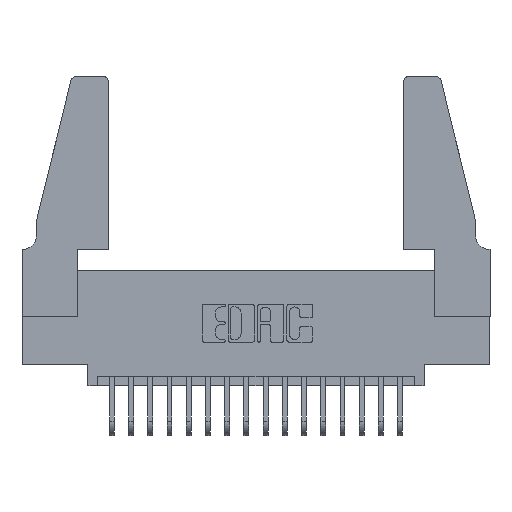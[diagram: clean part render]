
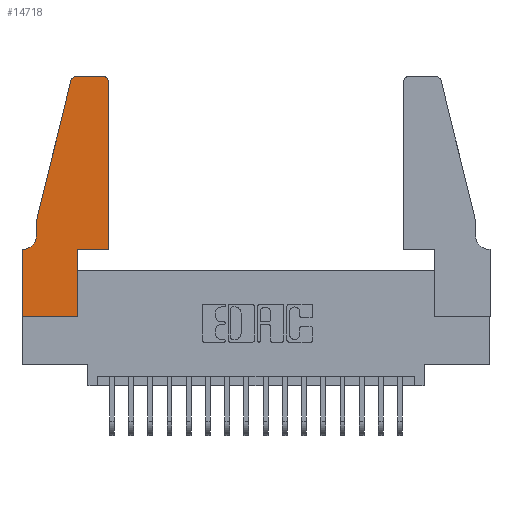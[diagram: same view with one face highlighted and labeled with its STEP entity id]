
A CAD part, top view. The second image highlights one B-rep face of the part: STEP entity #14718.
In plain terms, the highlighted planar face has unit normal (0, 0, 1).
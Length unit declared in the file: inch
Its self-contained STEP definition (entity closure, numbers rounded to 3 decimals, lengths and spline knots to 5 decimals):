
#206 = DIRECTION ( 'NONE',  ( 0., 0., -1. ) ) ;
#715 = VERTEX_POINT ( 'NONE', #1710 ) ;
#738 = DIRECTION ( 'NONE',  ( 1., 0., 0. ) ) ;
#847 = VERTEX_POINT ( 'NONE', #10963 ) ;
#925 = VECTOR ( 'NONE', #5029, 39.37008 ) ;
#1072 = CARTESIAN_POINT ( 'NONE',  ( 0.4205, 1.22, 0.37 ) ) ;
#1340 = DIRECTION ( 'NONE',  ( 0., 0., 1. ) ) ;
#1411 = VECTOR ( 'NONE', #2004, 39.37008 ) ;
#1440 = CARTESIAN_POINT ( 'NONE',  ( 0., 0., 0.37 ) ) ;
#1502 = CARTESIAN_POINT ( 'NONE',  ( 0., 0.35, 0.37 ) ) ;
#1572 = ORIENTED_EDGE ( 'NONE', *, *, #3822, .T. ) ;
#1633 = VERTEX_POINT ( 'NONE', #12237 ) ;
#1710 = CARTESIAN_POINT ( 'NONE',  ( 0., 0., 0.37 ) ) ;
#1793 = ORIENTED_EDGE ( 'NONE', *, *, #8181, .T. ) ;
#1916 = DIRECTION ( 'NONE',  ( -1., 0., 0. ) ) ;
#2004 = DIRECTION ( 'NONE',  ( -1., 0., 0. ) ) ;
#2450 = DIRECTION ( 'NONE',  ( 1., 0., 0. ) ) ;
#2582 = CIRCLE ( 'NONE', #15649, 0.03 ) ;
#2890 = VERTEX_POINT ( 'NONE', #16645 ) ;
#2892 = DIRECTION ( 'NONE',  ( 0., 0., 1. ) ) ;
#2964 = CARTESIAN_POINT ( 'NONE',  ( 0.0755, 0.5, 0.37 ) ) ;
#3071 = EDGE_CURVE ( 'NONE', #847, #4168, #12786, .T. ) ;
#3456 = AXIS2_PLACEMENT_3D ( 'NONE', #9681, #1340, #11104 ) ;
#3622 = ORIENTED_EDGE ( 'NONE', *, *, #13378, .T. ) ;
#3761 = EDGE_CURVE ( 'NONE', #17357, #17166, #5144, .T. ) ;
#3780 = ORIENTED_EDGE ( 'NONE', *, *, #17368, .T. ) ;
#3821 = VECTOR ( 'NONE', #738, 39.37008 ) ;
#3822 = EDGE_CURVE ( 'NONE', #715, #10002, #4244, .T. ) ;
#4168 = VERTEX_POINT ( 'NONE', #15318 ) ;
#4244 = LINE ( 'NONE', #10481, #3821 ) ;
#4632 = LINE ( 'NONE', #14744, #925 ) ;
#4639 = ORIENTED_EDGE ( 'NONE', *, *, #6131, .T. ) ;
#4774 = CARTESIAN_POINT ( 'NONE',  ( 0.2605, 1.25, 0.37 ) ) ;
#5029 = DIRECTION ( 'NONE',  ( 0., 1., 0. ) ) ;
#5113 = CARTESIAN_POINT ( 'NONE',  ( 0.0755, 0.5, 0.37 ) ) ;
#5144 = LINE ( 'NONE', #4774, #1411 ) ;
#5149 = ORIENTED_EDGE ( 'NONE', *, *, #5759, .T. ) ;
#5212 = CARTESIAN_POINT ( 'NONE',  ( 0.2865, 0., 0.37 ) ) ;
#5598 = CARTESIAN_POINT ( 'NONE',  ( 0.25487, 1.22718, 0.37 ) ) ;
#5705 = VERTEX_POINT ( 'NONE', #5598 ) ;
#5759 = EDGE_CURVE ( 'NONE', #4168, #715, #16313, .T. ) ;
#6038 = CARTESIAN_POINT ( 'NONE',  ( 0.4505, 0.35, 0.37 ) ) ;
#6131 = EDGE_CURVE ( 'NONE', #1633, #7313, #6620, .T. ) ;
#6490 = DIRECTION ( 'NONE',  ( 1., 0., 0. ) ) ;
#6620 = LINE ( 'NONE', #13445, #9873 ) ;
#7240 = ORIENTED_EDGE ( 'NONE', *, *, #9320, .T. ) ;
#7313 = VERTEX_POINT ( 'NONE', #16549 ) ;
#7434 = EDGE_CURVE ( 'NONE', #5705, #16830, #15043, .T. ) ;
#7519 = ORIENTED_EDGE ( 'NONE', *, *, #9559, .T. ) ;
#7585 = VECTOR ( 'NONE', #8404, 39.37008 ) ;
#8181 = EDGE_CURVE ( 'NONE', #7313, #11270, #17535, .T. ) ;
#8404 = DIRECTION ( 'NONE',  ( 0., -1., 0. ) ) ;
#8517 = CARTESIAN_POINT ( 'NONE',  ( 0.0055, 0.42, 0.37 ) ) ;
#9081 = ORIENTED_EDGE ( 'NONE', *, *, #10144, .T. ) ;
#9320 = EDGE_CURVE ( 'NONE', #11270, #17357, #2582, .T. ) ;
#9559 = EDGE_CURVE ( 'NONE', #2890, #847, #12201, .T. ) ;
#9681 = CARTESIAN_POINT ( 'NONE',  ( 0.284, 1.22, 0.37 ) ) ;
#9737 = AXIS2_PLACEMENT_3D ( 'NONE', #8517, #206, #9945 ) ;
#9842 = PLANE ( 'NONE',  #17424 ) ;
#9873 = VECTOR ( 'NONE', #6490, 39.37008 ) ;
#9945 = DIRECTION ( 'NONE',  ( -1., 0., 0. ) ) ;
#10002 = VERTEX_POINT ( 'NONE', #5212 ) ;
#10144 = EDGE_CURVE ( 'NONE', #17166, #5705, #14986, .T. ) ;
#10232 = DIRECTION ( 'NONE',  ( 0., 1., 0. ) ) ;
#10481 = CARTESIAN_POINT ( 'NONE',  ( 0., 0., 0.37 ) ) ;
#10763 = ORIENTED_EDGE ( 'NONE', *, *, #3071, .T. ) ;
#10821 = DIRECTION ( 'NONE',  ( 0., 0., 1. ) ) ;
#10963 = CARTESIAN_POINT ( 'NONE',  ( 0.0055, 0.35, 0.37 ) ) ;
#11104 = DIRECTION ( 'NONE',  ( 1., 0., 0. ) ) ;
#11270 = VERTEX_POINT ( 'NONE', #13610 ) ;
#11323 = DIRECTION ( 'NONE',  ( -0.239, -0.971, 0. ) ) ;
#11804 = VECTOR ( 'NONE', #11323, 39.37008 ) ;
#12201 = CIRCLE ( 'NONE', #9737, 0.07 ) ;
#12237 = CARTESIAN_POINT ( 'NONE',  ( 0.2865, 0.35, 0.37 ) ) ;
#12673 = DIRECTION ( 'NONE',  ( 1., 0., 0. ) ) ;
#12786 = LINE ( 'NONE', #15806, #16000 ) ;
#13039 = FACE_OUTER_BOUND ( 'NONE', #17294, .T. ) ;
#13378 = EDGE_CURVE ( 'NONE', #16830, #2890, #17724, .T. ) ;
#13445 = CARTESIAN_POINT ( 'NONE',  ( 0.4505, 0.35, 0.37 ) ) ;
#13610 = CARTESIAN_POINT ( 'NONE',  ( 0.4505, 1.22, 0.37 ) ) ;
#14057 = DIRECTION ( 'NONE',  ( 0., -1., 0. ) ) ;
#14167 = ORIENTED_EDGE ( 'NONE', *, *, #3761, .T. ) ;
#14718 = ADVANCED_FACE ( 'NONE', ( #13039 ), #9842, .T. ) ;
#14744 = CARTESIAN_POINT ( 'NONE',  ( 0.2865, 0.35, 0.37 ) ) ;
#14986 = CIRCLE ( 'NONE', #3456, 0.03 ) ;
#15043 = LINE ( 'NONE', #2964, #11804 ) ;
#15318 = CARTESIAN_POINT ( 'NONE',  ( 0., 0.35, 0.37 ) ) ;
#15649 = AXIS2_PLACEMENT_3D ( 'NONE', #1072, #10821, #2450 ) ;
#15684 = CARTESIAN_POINT ( 'NONE',  ( 0.284, 1.25, 0.37 ) ) ;
#15806 = CARTESIAN_POINT ( 'NONE',  ( 0.0755, 0.35, 0.37 ) ) ;
#15896 = VECTOR ( 'NONE', #14057, 39.37008 ) ;
#16000 = VECTOR ( 'NONE', #1916, 39.37008 ) ;
#16313 = LINE ( 'NONE', #1440, #15896 ) ;
#16549 = CARTESIAN_POINT ( 'NONE',  ( 0.4505, 0.35, 0.37 ) ) ;
#16623 = ORIENTED_EDGE ( 'NONE', *, *, #7434, .T. ) ;
#16645 = CARTESIAN_POINT ( 'NONE',  ( 0.0755, 0.42, 0.37 ) ) ;
#16710 = CARTESIAN_POINT ( 'NONE',  ( 0.0755, 0.5, 0.37 ) ) ;
#16830 = VERTEX_POINT ( 'NONE', #5113 ) ;
#17116 = VECTOR ( 'NONE', #10232, 39.37008 ) ;
#17166 = VERTEX_POINT ( 'NONE', #15684 ) ;
#17294 = EDGE_LOOP ( 'NONE', ( #14167, #9081, #16623, #3622, #7519, #10763, #5149, #1572, #3780, #4639, #1793, #7240 ) ) ;
#17357 = VERTEX_POINT ( 'NONE', #17456 ) ;
#17368 = EDGE_CURVE ( 'NONE', #10002, #1633, #4632, .T. ) ;
#17424 = AXIS2_PLACEMENT_3D ( 'NONE', #1502, #2892, #12673 ) ;
#17456 = CARTESIAN_POINT ( 'NONE',  ( 0.4205, 1.25, 0.37 ) ) ;
#17535 = LINE ( 'NONE', #6038, #17116 ) ;
#17724 = LINE ( 'NONE', #16710, #7585 ) ;
